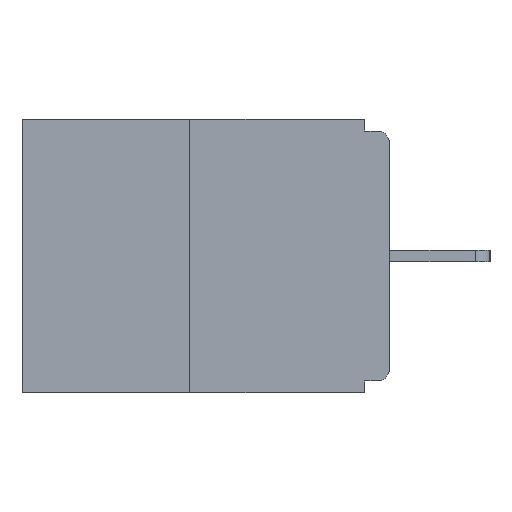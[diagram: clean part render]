
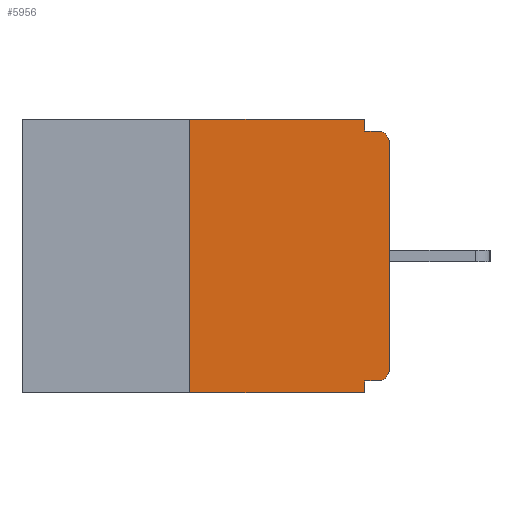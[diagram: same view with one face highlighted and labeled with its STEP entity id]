
A CAD part, left-side view. The second image highlights one B-rep face of the part: STEP entity #5956.
In plain terms, the highlighted planar face has unit normal (-1, 0, 0).
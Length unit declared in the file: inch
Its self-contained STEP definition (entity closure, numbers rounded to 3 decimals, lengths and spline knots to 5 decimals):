
#68 = CARTESIAN_POINT ( 'NONE',  ( 0., 0.015, -0.313 ) ) ;
#295 = VERTEX_POINT ( 'NONE', #5787 ) ;
#379 = EDGE_LOOP ( 'NONE', ( #12472, #4344, #16476, #6797, #629, #10427, #16822, #5303, #7599, #8964 ) ) ;
#629 = ORIENTED_EDGE ( 'NONE', *, *, #16206, .F. ) ;
#726 = VECTOR ( 'NONE', #7779, 39.37008 ) ;
#911 = VECTOR ( 'NONE', #3478, 39.37008 ) ;
#999 = VECTOR ( 'NONE', #14947, 39.37008 ) ;
#1393 = CIRCLE ( 'NONE', #3313, 0.015 ) ;
#1850 = VERTEX_POINT ( 'NONE', #16021 ) ;
#2009 = CARTESIAN_POINT ( 'NONE',  ( 0., 0., -0.03 ) ) ;
#2627 = VERTEX_POINT ( 'NONE', #8211 ) ;
#2725 = DIRECTION ( 'NONE',  ( -1., 0., 0. ) ) ;
#2766 = CARTESIAN_POINT ( 'NONE',  ( 0., 0.031, -0.328 ) ) ;
#3106 = CARTESIAN_POINT ( 'NONE',  ( 0., 0., -0.313 ) ) ;
#3116 = VERTEX_POINT ( 'NONE', #3106 ) ;
#3313 = AXIS2_PLACEMENT_3D ( 'NONE', #10492, #2725, #5157 ) ;
#3327 = AXIS2_PLACEMENT_3D ( 'NONE', #68, #4993, #3872 ) ;
#3366 = DIRECTION ( 'NONE',  ( 0., 0., -1. ) ) ;
#3478 = DIRECTION ( 'NONE',  ( 0., 0., -1. ) ) ;
#3864 = VERTEX_POINT ( 'NONE', #12454 ) ;
#3872 = DIRECTION ( 'NONE',  ( 0., 0., -1. ) ) ;
#4093 = LINE ( 'NONE', #12279, #14035 ) ;
#4344 = ORIENTED_EDGE ( 'NONE', *, *, #6736, .F. ) ;
#4446 = LINE ( 'NONE', #9716, #999 ) ;
#4535 = VECTOR ( 'NONE', #15089, 39.37008 ) ;
#4605 = CARTESIAN_POINT ( 'NONE',  ( 0., 0.25, 0. ) ) ;
#4682 = VECTOR ( 'NONE', #13227, 39.37008 ) ;
#4768 = EDGE_CURVE ( 'NONE', #3116, #6659, #10408, .T. ) ;
#4993 = DIRECTION ( 'NONE',  ( -1., 0., 0. ) ) ;
#5157 = DIRECTION ( 'NONE',  ( 0., 0., -1. ) ) ;
#5303 = ORIENTED_EDGE ( 'NONE', *, *, #11314, .T. ) ;
#5622 = VERTEX_POINT ( 'NONE', #2766 ) ;
#5720 = LINE ( 'NONE', #10975, #4682 ) ;
#5787 = CARTESIAN_POINT ( 'NONE',  ( 0., 0.031, -0.015 ) ) ;
#5956 = ADVANCED_FACE ( 'NONE', ( #12669 ), #14043, .F. ) ;
#6493 = EDGE_CURVE ( 'NONE', #295, #2627, #12019, .T. ) ;
#6659 = VERTEX_POINT ( 'NONE', #2009 ) ;
#6673 = DIRECTION ( 'NONE',  ( 0., -1., 0. ) ) ;
#6729 = VECTOR ( 'NONE', #7488, 39.37008 ) ;
#6736 = EDGE_CURVE ( 'NONE', #8032, #1850, #11155, .T. ) ;
#6797 = ORIENTED_EDGE ( 'NONE', *, *, #15442, .F. ) ;
#7488 = DIRECTION ( 'NONE',  ( 0., 0., 1. ) ) ;
#7529 = CARTESIAN_POINT ( 'NONE',  ( 0., 0.031, -0.343 ) ) ;
#7599 = ORIENTED_EDGE ( 'NONE', *, *, #6493, .F. ) ;
#7779 = DIRECTION ( 'NONE',  ( 0., 0., -1. ) ) ;
#7828 = CARTESIAN_POINT ( 'NONE',  ( 0., 0., 0. ) ) ;
#7840 = VECTOR ( 'NONE', #6673, 39.37008 ) ;
#8032 = VERTEX_POINT ( 'NONE', #13274 ) ;
#8211 = CARTESIAN_POINT ( 'NONE',  ( 0., 0.015, -0.015 ) ) ;
#8459 = CARTESIAN_POINT ( 'NONE',  ( 0., 0.031, -0.343 ) ) ;
#8964 = ORIENTED_EDGE ( 'NONE', *, *, #10384, .F. ) ;
#9387 = CIRCLE ( 'NONE', #3327, 0.015 ) ;
#9716 = CARTESIAN_POINT ( 'NONE',  ( 0., 0.46, 0. ) ) ;
#10029 = AXIS2_PLACEMENT_3D ( 'NONE', #12761, #13882, #3366 ) ;
#10273 = LINE ( 'NONE', #16987, #726 ) ;
#10278 = EDGE_CURVE ( 'NONE', #1850, #3864, #4446, .T. ) ;
#10384 = EDGE_CURVE ( 'NONE', #3864, #295, #10273, .T. ) ;
#10395 = VERTEX_POINT ( 'NONE', #14236 ) ;
#10408 = LINE ( 'NONE', #7828, #6729 ) ;
#10427 = ORIENTED_EDGE ( 'NONE', *, *, #11497, .T. ) ;
#10492 = CARTESIAN_POINT ( 'NONE',  ( 0., 0.015, -0.03 ) ) ;
#10975 = CARTESIAN_POINT ( 'NONE',  ( 0., 0.46, -0.343 ) ) ;
#11155 = LINE ( 'NONE', #4605, #4535 ) ;
#11314 = EDGE_CURVE ( 'NONE', #6659, #2627, #1393, .T. ) ;
#11497 = EDGE_CURVE ( 'NONE', #10395, #3116, #9387, .T. ) ;
#11938 = CARTESIAN_POINT ( 'NONE',  ( 0., 0., -0.015 ) ) ;
#12019 = LINE ( 'NONE', #11938, #7840 ) ;
#12279 = CARTESIAN_POINT ( 'NONE',  ( 0., 0., -0.328 ) ) ;
#12454 = CARTESIAN_POINT ( 'NONE',  ( 0., 0.031, 0. ) ) ;
#12472 = ORIENTED_EDGE ( 'NONE', *, *, #10278, .F. ) ;
#12529 = LINE ( 'NONE', #7529, #911 ) ;
#12669 = FACE_OUTER_BOUND ( 'NONE', #379, .T. ) ;
#12761 = CARTESIAN_POINT ( 'NONE',  ( 0., 0.46, 0. ) ) ;
#13227 = DIRECTION ( 'NONE',  ( 0., -1., 0. ) ) ;
#13274 = CARTESIAN_POINT ( 'NONE',  ( 0., 0.25, -0.343 ) ) ;
#13316 = DIRECTION ( 'NONE',  ( 0., 1., 0. ) ) ;
#13882 = DIRECTION ( 'NONE',  ( 1., 0., 0. ) ) ;
#14035 = VECTOR ( 'NONE', #13316, 39.37008 ) ;
#14043 = PLANE ( 'NONE',  #10029 ) ;
#14236 = CARTESIAN_POINT ( 'NONE',  ( 0., 0.015, -0.328 ) ) ;
#14947 = DIRECTION ( 'NONE',  ( 0., -1., 0. ) ) ;
#15089 = DIRECTION ( 'NONE',  ( 0., 0., 1. ) ) ;
#15442 = EDGE_CURVE ( 'NONE', #5622, #16936, #12529, .T. ) ;
#16021 = CARTESIAN_POINT ( 'NONE',  ( 0., 0.25, 0. ) ) ;
#16206 = EDGE_CURVE ( 'NONE', #10395, #5622, #4093, .T. ) ;
#16303 = EDGE_CURVE ( 'NONE', #8032, #16936, #5720, .T. ) ;
#16476 = ORIENTED_EDGE ( 'NONE', *, *, #16303, .T. ) ;
#16822 = ORIENTED_EDGE ( 'NONE', *, *, #4768, .T. ) ;
#16936 = VERTEX_POINT ( 'NONE', #8459 ) ;
#16987 = CARTESIAN_POINT ( 'NONE',  ( 0., 0.031, 0. ) ) ;
